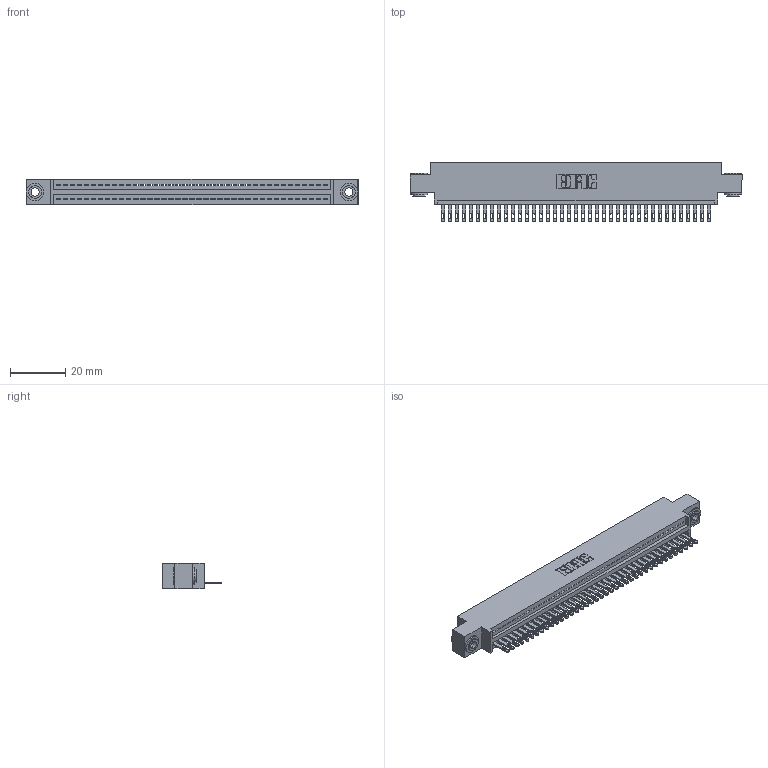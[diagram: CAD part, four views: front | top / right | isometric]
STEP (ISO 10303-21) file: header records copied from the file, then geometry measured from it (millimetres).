
FILE_DESCRIPTION (( 'STEP AP203' ), '1' );
FILE_NAME ('895-039-500-603.STEP', '2020-09-26T02:18:11', ( '' ), ( '' ), 'SwSTEP 2.0', 'SolidWorks 2020', '' );
FILE_SCHEMA (( 'CONFIG_CONTROL_DESIGN' ));
Length unit declared in the file: inch
Products named in the file (4): 345-292-001_345-293-100; 895-039-500-603; 845 Part_0.170 Offset - 0.156 Dia-TH; 345-250-002_345-250-002-102
Assembly tree (42 placements, depth 2):
  895-039-500-603
    845 Part_0.170 Offset - 0.156 Dia-TH
    345-292-001_345-293-100  x39
    345-250-002_345-250-002-102  x2
Bounding box: 120.27 x 21.51 x 9.4 mm (x, y, z)
Volume: 11328.8 mm3; surface area: 15442.9 mm2
Topology: 42 solids, 42 shells, 2274 faces, 6981 edges, 4650 vertices
Faces by surface type: plane 1420, cylinder 846, cone 8
Entity records: 30468 total; most frequent: CARTESIAN_POINT 5256, ORIENTED_EDGE 5222, DIRECTION 4627, EDGE_CURVE 2611, LINE 2295, VECTOR 2295, VERTEX_POINT 1738, AXIS2_PLACEMENT_3D 1166
